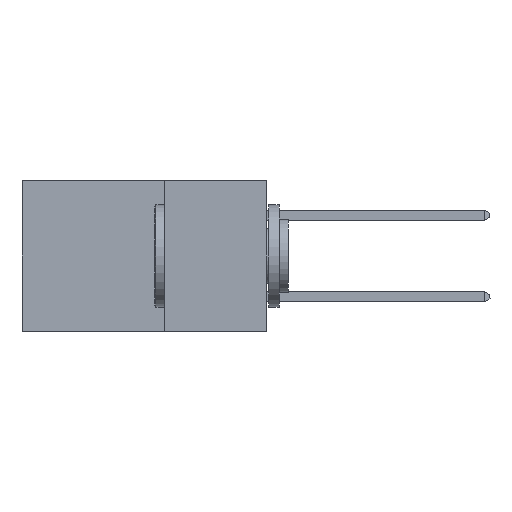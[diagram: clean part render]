
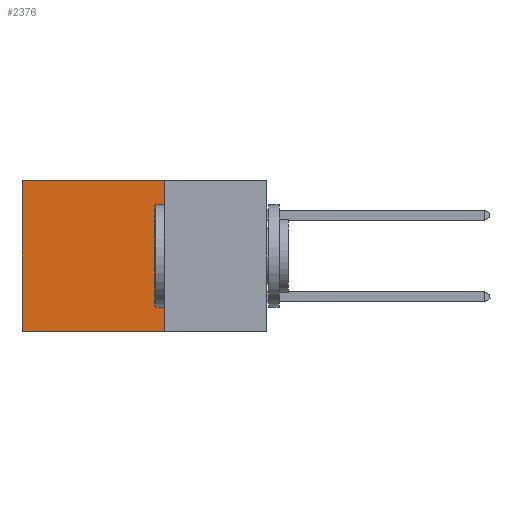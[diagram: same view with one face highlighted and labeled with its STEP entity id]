
A CAD part, left-side view. The second image highlights one B-rep face of the part: STEP entity #2376.
In plain terms, the highlighted planar face has unit normal (-1, 0, 0).
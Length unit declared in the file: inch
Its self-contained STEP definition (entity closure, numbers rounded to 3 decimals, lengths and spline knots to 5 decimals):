
#562 = EDGE_CURVE ( 'NONE', #21123, #11431, #11023, .T. ) ;
#1292 = CARTESIAN_POINT ( 'NONE',  ( 0.2875, 0.6, 0. ) ) ;
#1747 = CARTESIAN_POINT ( 'NONE',  ( 0.2875, 0.25, 0. ) ) ;
#2376 = ADVANCED_FACE ( 'NONE', ( #4591 ), #13011, .F. ) ;
#2965 = DIRECTION ( 'NONE',  ( 0., 0., -1. ) ) ;
#3456 = DIRECTION ( 'NONE',  ( 0., 1., 0. ) ) ;
#3864 = LINE ( 'NONE', #1747, #7941 ) ;
#4591 = FACE_OUTER_BOUND ( 'NONE', #12908, .T. ) ;
#6240 = VERTEX_POINT ( 'NONE', #21456 ) ;
#6930 = CARTESIAN_POINT ( 'NONE',  ( 0.2875, 0.25, -0.37 ) ) ;
#7941 = VECTOR ( 'NONE', #3456, 39.37008 ) ;
#8790 = VECTOR ( 'NONE', #13581, 39.37008 ) ;
#9480 = LINE ( 'NONE', #20835, #13590 ) ;
#9737 = ORIENTED_EDGE ( 'NONE', *, *, #17151, .T. ) ;
#10153 = ORIENTED_EDGE ( 'NONE', *, *, #19815, .F. ) ;
#10423 = ORIENTED_EDGE ( 'NONE', *, *, #562, .F. ) ;
#10452 = CARTESIAN_POINT ( 'NONE',  ( 0.2875, 0.6, 0. ) ) ;
#10463 = VECTOR ( 'NONE', #2965, 39.37008 ) ;
#11023 = LINE ( 'NONE', #13853, #10463 ) ;
#11066 = ORIENTED_EDGE ( 'NONE', *, *, #17345, .T. ) ;
#11431 = VERTEX_POINT ( 'NONE', #6930 ) ;
#12350 = DIRECTION ( 'NONE',  ( 0., 0., -1. ) ) ;
#12399 = DIRECTION ( 'NONE',  ( 0., 1., 0. ) ) ;
#12694 = DIRECTION ( 'NONE',  ( 1., 0., 0. ) ) ;
#12908 = EDGE_LOOP ( 'NONE', ( #9737, #10153, #10423, #11066 ) ) ;
#13011 = PLANE ( 'NONE',  #14583 ) ;
#13581 = DIRECTION ( 'NONE',  ( 0., 0., -1. ) ) ;
#13590 = VECTOR ( 'NONE', #12399, 39.37008 ) ;
#13853 = CARTESIAN_POINT ( 'NONE',  ( 0.2875, 0.25, 0. ) ) ;
#13996 = CARTESIAN_POINT ( 'NONE',  ( 0.2875, 0.25, 0. ) ) ;
#14174 = VERTEX_POINT ( 'NONE', #10452 ) ;
#14583 = AXIS2_PLACEMENT_3D ( 'NONE', #13996, #12694, #12350 ) ;
#16420 = LINE ( 'NONE', #1292, #8790 ) ;
#17151 = EDGE_CURVE ( 'NONE', #14174, #6240, #16420, .T. ) ;
#17345 = EDGE_CURVE ( 'NONE', #21123, #14174, #3864, .T. ) ;
#19378 = CARTESIAN_POINT ( 'NONE',  ( 0.2875, 0.25, 0. ) ) ;
#19815 = EDGE_CURVE ( 'NONE', #11431, #6240, #9480, .T. ) ;
#20835 = CARTESIAN_POINT ( 'NONE',  ( 0.2875, 0.25, -0.37 ) ) ;
#21123 = VERTEX_POINT ( 'NONE', #19378 ) ;
#21456 = CARTESIAN_POINT ( 'NONE',  ( 0.2875, 0.6, -0.37 ) ) ;
